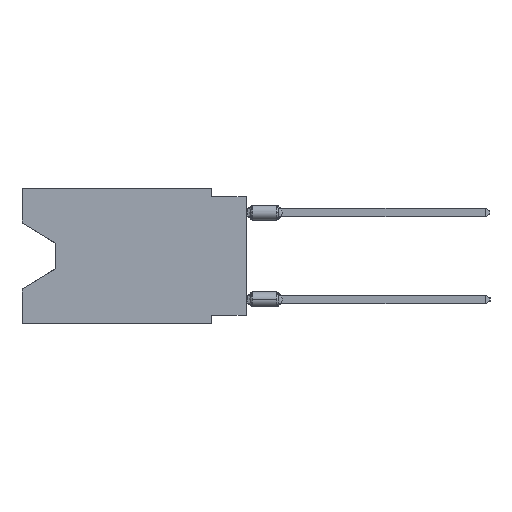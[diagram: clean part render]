
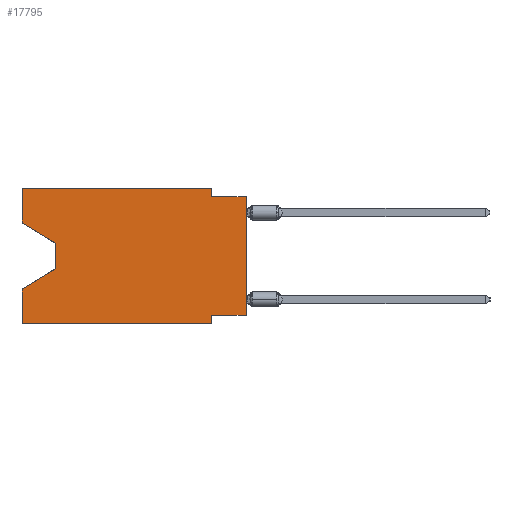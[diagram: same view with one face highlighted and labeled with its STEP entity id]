
A CAD part, left-side view. The second image highlights one B-rep face of the part: STEP entity #17795.
In plain terms, the highlighted planar face has unit normal (-1, 0, 0).
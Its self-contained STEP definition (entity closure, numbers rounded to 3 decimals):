
#542 = LINE ( 'NONE', #37822, #12198 ) ;
#992 = DIRECTION ( 'NONE',  ( 0., -1., 0. ) ) ;
#1359 = CARTESIAN_POINT ( 'NONE',  ( 0., 16.383, -7.36 ) ) ;
#1513 = VERTEX_POINT ( 'NONE', #16368 ) ;
#2015 = ORIENTED_EDGE ( 'NONE', *, *, #36327, .F. ) ;
#2043 = VERTEX_POINT ( 'NONE', #4552 ) ;
#2298 = AXIS2_PLACEMENT_3D ( 'NONE', #30248, #40486, #24697 ) ;
#2313 = LINE ( 'NONE', #13149, #40954 ) ;
#2735 = DIRECTION ( 'NONE',  ( 0., 1., 0. ) ) ;
#2747 = ORIENTED_EDGE ( 'NONE', *, *, #29237, .T. ) ;
#3020 = EDGE_LOOP ( 'NONE', ( #28398, #6561, #3088, #24764, #2747, #18022, #2015, #24453, #7619, #26063, #30973, #21830 ) ) ;
#3088 = ORIENTED_EDGE ( 'NONE', *, *, #20600, .T. ) ;
#3220 = FACE_OUTER_BOUND ( 'NONE', #3020, .T. ) ;
#3528 = VERTEX_POINT ( 'NONE', #40026 ) ;
#3601 = VECTOR ( 'NONE', #32154, 1000. ) ;
#3602 = VECTOR ( 'NONE', #42446, 1000. ) ;
#3846 = EDGE_CURVE ( 'NONE', #11449, #27031, #24265, .T. ) ;
#4306 = VERTEX_POINT ( 'NONE', #1359 ) ;
#4552 = CARTESIAN_POINT ( 'NONE',  ( 0., 13.97, -4.013 ) ) ;
#5320 = EDGE_CURVE ( 'NONE', #1513, #3528, #22259, .T. ) ;
#6223 = CARTESIAN_POINT ( 'NONE',  ( 0., 13.97, -5.893 ) ) ;
#6245 = CARTESIAN_POINT ( 'NONE',  ( 0., 2.54, -0.635 ) ) ;
#6561 = ORIENTED_EDGE ( 'NONE', *, *, #38250, .T. ) ;
#6782 = CARTESIAN_POINT ( 'NONE',  ( 0., 16.383, -2.546 ) ) ;
#6977 = CARTESIAN_POINT ( 'NONE',  ( 0., 16.383, -2.546 ) ) ;
#6986 = DIRECTION ( 'NONE',  ( 0., -0.855, -0.519 ) ) ;
#7218 = DIRECTION ( 'NONE',  ( 0., 0., 1. ) ) ;
#7619 = ORIENTED_EDGE ( 'NONE', *, *, #3846, .F. ) ;
#8419 = DIRECTION ( 'NONE',  ( 0., 0., 1. ) ) ;
#9814 = VECTOR ( 'NONE', #6986, 1000. ) ;
#10185 = CARTESIAN_POINT ( 'NONE',  ( 0., 16.383, 0. ) ) ;
#10958 = CARTESIAN_POINT ( 'NONE',  ( 0., 0., -0.635 ) ) ;
#11449 = VERTEX_POINT ( 'NONE', #6245 ) ;
#11960 = VECTOR ( 'NONE', #992, 1000. ) ;
#12198 = VECTOR ( 'NONE', #7218, 1000. ) ;
#12303 = LINE ( 'NONE', #35809, #13943 ) ;
#13149 = CARTESIAN_POINT ( 'NONE',  ( 0., 0., -9.271 ) ) ;
#13943 = VECTOR ( 'NONE', #24954, 1000. ) ;
#13999 = CARTESIAN_POINT ( 'NONE',  ( 0., 2.54, -9.906 ) ) ;
#15089 = CARTESIAN_POINT ( 'NONE',  ( 0., 13.97, -4.013 ) ) ;
#16244 = CARTESIAN_POINT ( 'NONE',  ( 0., 16.383, 0. ) ) ;
#16368 = CARTESIAN_POINT ( 'NONE',  ( 0., 16.383, 0. ) ) ;
#16394 = CARTESIAN_POINT ( 'NONE',  ( 0., 2.54, -9.271 ) ) ;
#17795 = ADVANCED_FACE ( 'NONE', ( #3220 ), #26942, .F. ) ;
#18022 = ORIENTED_EDGE ( 'NONE', *, *, #35259, .F. ) ;
#19013 = EDGE_CURVE ( 'NONE', #3528, #11449, #34318, .T. ) ;
#19144 = LINE ( 'NONE', #35604, #3602 ) ;
#19686 = VERTEX_POINT ( 'NONE', #41527 ) ;
#20600 = EDGE_CURVE ( 'NONE', #33736, #4306, #19144, .T. ) ;
#21451 = EDGE_CURVE ( 'NONE', #36519, #27031, #42139, .T. ) ;
#21568 = VERTEX_POINT ( 'NONE', #16394 ) ;
#21830 = ORIENTED_EDGE ( 'NONE', *, *, #33371, .F. ) ;
#22259 = LINE ( 'NONE', #16244, #32412 ) ;
#22377 = CARTESIAN_POINT ( 'NONE',  ( 0., 0., 0. ) ) ;
#22745 = VECTOR ( 'NONE', #8419, 1000. ) ;
#24054 = LINE ( 'NONE', #6782, #9814 ) ;
#24258 = EDGE_CURVE ( 'NONE', #33411, #2043, #24054, .T. ) ;
#24265 = LINE ( 'NONE', #10958, #11960 ) ;
#24453 = ORIENTED_EDGE ( 'NONE', *, *, #21451, .T. ) ;
#24697 = DIRECTION ( 'NONE',  ( 0., 0., -1. ) ) ;
#24764 = ORIENTED_EDGE ( 'NONE', *, *, #42359, .F. ) ;
#24954 = DIRECTION ( 'NONE',  ( 0., -1., 0. ) ) ;
#24968 = VECTOR ( 'NONE', #27241, 1000. ) ;
#25057 = LINE ( 'NONE', #15089, #3601 ) ;
#26063 = ORIENTED_EDGE ( 'NONE', *, *, #19013, .F. ) ;
#26334 = VECTOR ( 'NONE', #27523, 1000. ) ;
#26942 = PLANE ( 'NONE',  #2298 ) ;
#27031 = VERTEX_POINT ( 'NONE', #34839 ) ;
#27241 = DIRECTION ( 'NONE',  ( 0., 0., 1. ) ) ;
#27523 = DIRECTION ( 'NONE',  ( 0., 0., -1. ) ) ;
#28394 = VECTOR ( 'NONE', #40546, 1000. ) ;
#28398 = ORIENTED_EDGE ( 'NONE', *, *, #24258, .T. ) ;
#29237 = EDGE_CURVE ( 'NONE', #19686, #36862, #12303, .T. ) ;
#30107 = CARTESIAN_POINT ( 'NONE',  ( 0., 2.54, 0. ) ) ;
#30248 = CARTESIAN_POINT ( 'NONE',  ( 0., 16.383, 0. ) ) ;
#30973 = ORIENTED_EDGE ( 'NONE', *, *, #5320, .F. ) ;
#31331 = CARTESIAN_POINT ( 'NONE',  ( 0., 0., -9.271 ) ) ;
#32154 = DIRECTION ( 'NONE',  ( 0., 0., -1. ) ) ;
#32412 = VECTOR ( 'NONE', #35992, 1000. ) ;
#33371 = EDGE_CURVE ( 'NONE', #33411, #1513, #542, .T. ) ;
#33411 = VERTEX_POINT ( 'NONE', #6977 ) ;
#33736 = VERTEX_POINT ( 'NONE', #6223 ) ;
#34318 = LINE ( 'NONE', #30107, #28394 ) ;
#34839 = CARTESIAN_POINT ( 'NONE',  ( 0., 0., -0.635 ) ) ;
#35259 = EDGE_CURVE ( 'NONE', #21568, #36862, #40192, .T. ) ;
#35604 = CARTESIAN_POINT ( 'NONE',  ( 0., 13.97, -5.893 ) ) ;
#35809 = CARTESIAN_POINT ( 'NONE',  ( 0., 16.383, -9.906 ) ) ;
#35992 = DIRECTION ( 'NONE',  ( 0., -1., 0. ) ) ;
#36327 = EDGE_CURVE ( 'NONE', #36519, #21568, #2313, .T. ) ;
#36519 = VERTEX_POINT ( 'NONE', #31331 ) ;
#36862 = VERTEX_POINT ( 'NONE', #37062 ) ;
#37062 = CARTESIAN_POINT ( 'NONE',  ( 0., 2.54, -9.906 ) ) ;
#37822 = CARTESIAN_POINT ( 'NONE',  ( 0., 16.383, 0. ) ) ;
#38250 = EDGE_CURVE ( 'NONE', #2043, #33736, #25057, .T. ) ;
#40026 = CARTESIAN_POINT ( 'NONE',  ( 0., 2.54, 0. ) ) ;
#40192 = LINE ( 'NONE', #13999, #26334 ) ;
#40486 = DIRECTION ( 'NONE',  ( 1., 0., 0. ) ) ;
#40546 = DIRECTION ( 'NONE',  ( 0., 0., -1. ) ) ;
#40574 = LINE ( 'NONE', #10185, #24968 ) ;
#40954 = VECTOR ( 'NONE', #2735, 1000. ) ;
#41527 = CARTESIAN_POINT ( 'NONE',  ( 0., 16.383, -9.906 ) ) ;
#42139 = LINE ( 'NONE', #22377, #22745 ) ;
#42359 = EDGE_CURVE ( 'NONE', #19686, #4306, #40574, .T. ) ;
#42446 = DIRECTION ( 'NONE',  ( 0., 0.855, -0.519 ) ) ;
